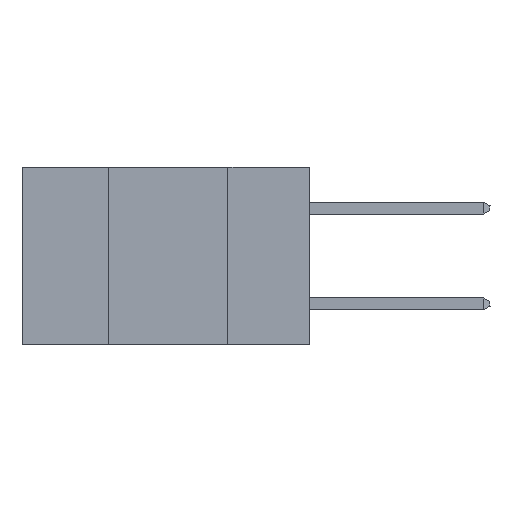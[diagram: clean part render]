
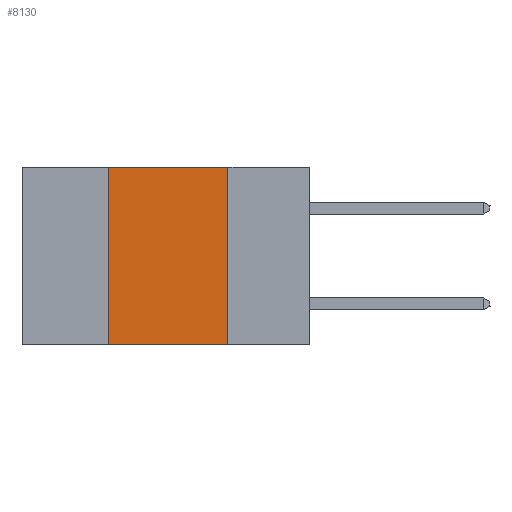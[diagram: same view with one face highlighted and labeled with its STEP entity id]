
A CAD part, left-side view. The second image highlights one B-rep face of the part: STEP entity #8130.
In plain terms, the highlighted planar face has unit normal (-1, 0, 0).
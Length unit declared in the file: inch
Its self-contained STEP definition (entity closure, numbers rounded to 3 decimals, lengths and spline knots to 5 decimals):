
#1136 = ORIENTED_EDGE ( 'NONE', *, *, #13824, .F. ) ;
#1827 = VERTEX_POINT ( 'NONE', #7105 ) ;
#2152 = DIRECTION ( 'NONE',  ( 0., 0., 1. ) ) ;
#3088 = AXIS2_PLACEMENT_3D ( 'NONE', #17071, #39707, #32156 ) ;
#4348 = DIRECTION ( 'NONE',  ( 0., 0., -1. ) ) ;
#5318 = CARTESIAN_POINT ( 'NONE',  ( 0., 0.17, 0. ) ) ;
#5953 = ORIENTED_EDGE ( 'NONE', *, *, #16946, .F. ) ;
#6316 = ORIENTED_EDGE ( 'NONE', *, *, #43306, .T. ) ;
#7105 = CARTESIAN_POINT ( 'NONE',  ( 0., 0.42, -0.37 ) ) ;
#8130 = ADVANCED_FACE ( 'NONE', ( #34902 ), #42705, .F. ) ;
#12896 = VERTEX_POINT ( 'NONE', #15872 ) ;
#13824 = EDGE_CURVE ( 'NONE', #12896, #28583, #39035, .T. ) ;
#15611 = VECTOR ( 'NONE', #2152, 39.37008 ) ;
#15872 = CARTESIAN_POINT ( 'NONE',  ( 0., 0.42, 0. ) ) ;
#16946 = EDGE_CURVE ( 'NONE', #1827, #12896, #33666, .T. ) ;
#17071 = CARTESIAN_POINT ( 'NONE',  ( 0., 0.6, 0. ) ) ;
#19374 = VECTOR ( 'NONE', #4348, 39.37008 ) ;
#22514 = EDGE_LOOP ( 'NONE', ( #34891, #1136, #5953, #6316 ) ) ;
#23829 = VECTOR ( 'NONE', #39879, 39.37008 ) ;
#26542 = CARTESIAN_POINT ( 'NONE',  ( 0., 0.17, -0.37 ) ) ;
#28583 = VERTEX_POINT ( 'NONE', #5318 ) ;
#29545 = DIRECTION ( 'NONE',  ( 0., -1., 0. ) ) ;
#31219 = LINE ( 'NONE', #33059, #19374 ) ;
#32156 = DIRECTION ( 'NONE',  ( 0., 0., -1. ) ) ;
#33059 = CARTESIAN_POINT ( 'NONE',  ( 0., 0.17, 0. ) ) ;
#33666 = LINE ( 'NONE', #41723, #15611 ) ;
#34891 = ORIENTED_EDGE ( 'NONE', *, *, #36883, .F. ) ;
#34902 = FACE_OUTER_BOUND ( 'NONE', #22514, .T. ) ;
#35920 = LINE ( 'NONE', #37220, #46608 ) ;
#36883 = EDGE_CURVE ( 'NONE', #28583, #43520, #31219, .T. ) ;
#37220 = CARTESIAN_POINT ( 'NONE',  ( 0., 0.6, -0.37 ) ) ;
#39035 = LINE ( 'NONE', #39722, #23829 ) ;
#39707 = DIRECTION ( 'NONE',  ( 1., 0., 0. ) ) ;
#39722 = CARTESIAN_POINT ( 'NONE',  ( 0., 0.6, 0. ) ) ;
#39879 = DIRECTION ( 'NONE',  ( 0., -1., 0. ) ) ;
#41723 = CARTESIAN_POINT ( 'NONE',  ( 0., 0.42, 0. ) ) ;
#42705 = PLANE ( 'NONE',  #3088 ) ;
#43306 = EDGE_CURVE ( 'NONE', #1827, #43520, #35920, .T. ) ;
#43520 = VERTEX_POINT ( 'NONE', #26542 ) ;
#46608 = VECTOR ( 'NONE', #29545, 39.37008 ) ;
